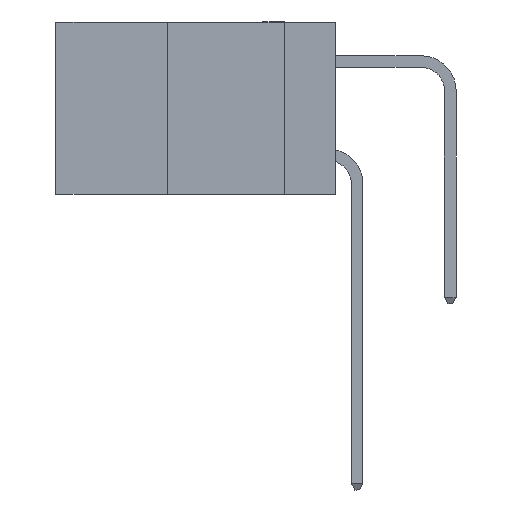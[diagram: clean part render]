
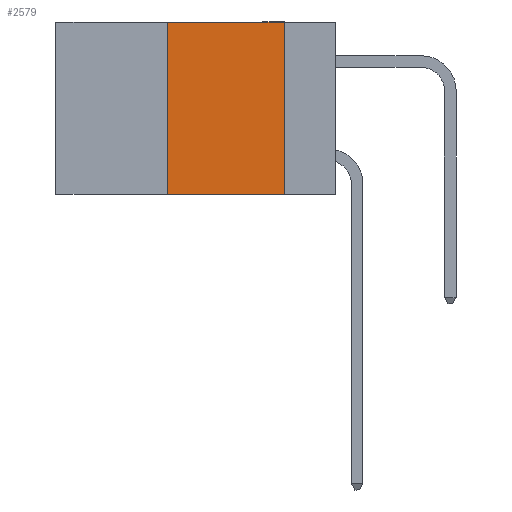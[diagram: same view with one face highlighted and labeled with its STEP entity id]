
A CAD part, left-side view. The second image highlights one B-rep face of the part: STEP entity #2579.
In plain terms, the highlighted planar face has unit normal (-1, 0, 0).
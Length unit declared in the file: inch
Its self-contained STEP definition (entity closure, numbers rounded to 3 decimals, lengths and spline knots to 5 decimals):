
#230 = CARTESIAN_POINT ( 'NONE',  ( 0., 0.36, -0.37 ) ) ;
#797 = CARTESIAN_POINT ( 'NONE',  ( 0., 0.6, 0. ) ) ;
#1622 = FACE_OUTER_BOUND ( 'NONE', #14554, .T. ) ;
#2401 = VECTOR ( 'NONE', #15415, 39.37008 ) ;
#2579 = ADVANCED_FACE ( 'NONE', ( #1622 ), #5075, .F. ) ;
#2629 = LINE ( 'NONE', #12782, #14123 ) ;
#2829 = ORIENTED_EDGE ( 'NONE', *, *, #14494, .F. ) ;
#3795 = DIRECTION ( 'NONE',  ( 0., 0., -1. ) ) ;
#4269 = CARTESIAN_POINT ( 'NONE',  ( 0., 0.11, -0.37 ) ) ;
#4716 = EDGE_CURVE ( 'NONE', #17787, #8776, #6358, .T. ) ;
#4803 = CARTESIAN_POINT ( 'NONE',  ( 0., 0.11, 0. ) ) ;
#5075 = PLANE ( 'NONE',  #5265 ) ;
#5265 = AXIS2_PLACEMENT_3D ( 'NONE', #797, #15769, #3795 ) ;
#6358 = LINE ( 'NONE', #16361, #14349 ) ;
#6527 = VECTOR ( 'NONE', #16015, 39.37008 ) ;
#8290 = DIRECTION ( 'NONE',  ( 0., -1., 0. ) ) ;
#8776 = VERTEX_POINT ( 'NONE', #4803 ) ;
#8816 = CARTESIAN_POINT ( 'NONE',  ( 0., 0.36, 0. ) ) ;
#8956 = ORIENTED_EDGE ( 'NONE', *, *, #10370, .T. ) ;
#10370 = EDGE_CURVE ( 'NONE', #14223, #16506, #18417, .T. ) ;
#12483 = LINE ( 'NONE', #8816, #2401 ) ;
#12782 = CARTESIAN_POINT ( 'NONE',  ( 0., 0.11, 0. ) ) ;
#13173 = ORIENTED_EDGE ( 'NONE', *, *, #15928, .F. ) ;
#14121 = ORIENTED_EDGE ( 'NONE', *, *, #4716, .F. ) ;
#14123 = VECTOR ( 'NONE', #15700, 39.37008 ) ;
#14223 = VERTEX_POINT ( 'NONE', #230 ) ;
#14349 = VECTOR ( 'NONE', #8290, 39.37008 ) ;
#14405 = CARTESIAN_POINT ( 'NONE',  ( 0., 0.36, 0. ) ) ;
#14494 = EDGE_CURVE ( 'NONE', #8776, #16506, #2629, .T. ) ;
#14540 = CARTESIAN_POINT ( 'NONE',  ( 0., 0.6, -0.37 ) ) ;
#14554 = EDGE_LOOP ( 'NONE', ( #2829, #14121, #13173, #8956 ) ) ;
#15415 = DIRECTION ( 'NONE',  ( 0., 0., 1. ) ) ;
#15700 = DIRECTION ( 'NONE',  ( 0., 0., -1. ) ) ;
#15769 = DIRECTION ( 'NONE',  ( 1., 0., 0. ) ) ;
#15928 = EDGE_CURVE ( 'NONE', #14223, #17787, #12483, .T. ) ;
#16015 = DIRECTION ( 'NONE',  ( 0., -1., 0. ) ) ;
#16361 = CARTESIAN_POINT ( 'NONE',  ( 0., 0.6, 0. ) ) ;
#16506 = VERTEX_POINT ( 'NONE', #4269 ) ;
#17787 = VERTEX_POINT ( 'NONE', #14405 ) ;
#18417 = LINE ( 'NONE', #14540, #6527 ) ;
